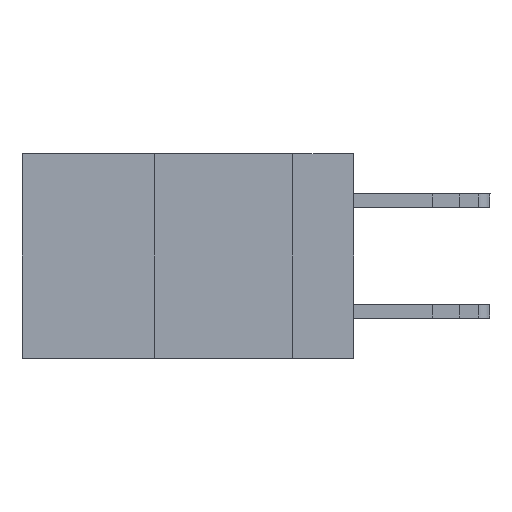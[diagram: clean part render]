
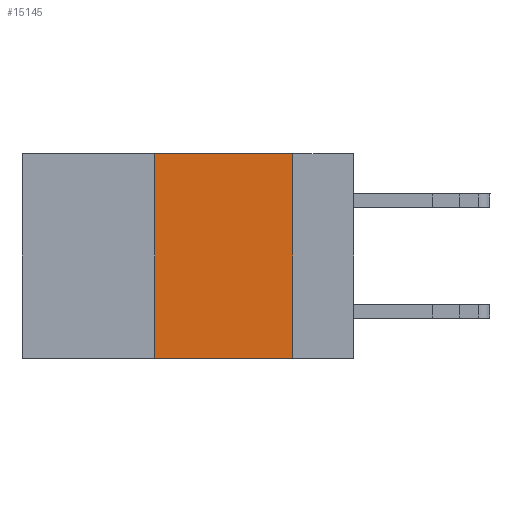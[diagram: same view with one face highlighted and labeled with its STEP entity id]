
A CAD part, left-side view. The second image highlights one B-rep face of the part: STEP entity #15145.
In plain terms, the highlighted planar face has unit normal (-1, 0, 0).
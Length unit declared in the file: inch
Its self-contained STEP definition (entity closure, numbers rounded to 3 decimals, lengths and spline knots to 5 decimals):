
#820 = DIRECTION ( 'NONE',  ( 0., 0., -1. ) ) ;
#977 = CARTESIAN_POINT ( 'NONE',  ( 0., 0.11, 0. ) ) ;
#1114 = VERTEX_POINT ( 'NONE', #13516 ) ;
#1533 = LINE ( 'NONE', #15673, #16303 ) ;
#2471 = CARTESIAN_POINT ( 'NONE',  ( 0., 0.6, -0.37 ) ) ;
#3147 = LINE ( 'NONE', #15863, #15089 ) ;
#6075 = ORIENTED_EDGE ( 'NONE', *, *, #16680, .F. ) ;
#6268 = FACE_OUTER_BOUND ( 'NONE', #8797, .T. ) ;
#7765 = VECTOR ( 'NONE', #22078, 39.37008 ) ;
#8781 = ORIENTED_EDGE ( 'NONE', *, *, #11999, .F. ) ;
#8797 = EDGE_LOOP ( 'NONE', ( #8781, #6075, #22035, #15753 ) ) ;
#9695 = VERTEX_POINT ( 'NONE', #977 ) ;
#10950 = LINE ( 'NONE', #2471, #13318 ) ;
#11747 = DIRECTION ( 'NONE',  ( 0., -1., 0. ) ) ;
#11999 = EDGE_CURVE ( 'NONE', #9695, #12107, #13712, .T. ) ;
#12107 = VERTEX_POINT ( 'NONE', #17070 ) ;
#13318 = VECTOR ( 'NONE', #16484, 39.37008 ) ;
#13516 = CARTESIAN_POINT ( 'NONE',  ( 0., 0.36, 0. ) ) ;
#13642 = VERTEX_POINT ( 'NONE', #20904 ) ;
#13712 = LINE ( 'NONE', #18902, #7765 ) ;
#14265 = EDGE_CURVE ( 'NONE', #13642, #1114, #3147, .T. ) ;
#14950 = DIRECTION ( 'NONE',  ( 1., 0., 0. ) ) ;
#15089 = VECTOR ( 'NONE', #16338, 39.37008 ) ;
#15126 = AXIS2_PLACEMENT_3D ( 'NONE', #16346, #14950, #820 ) ;
#15145 = ADVANCED_FACE ( 'NONE', ( #6268 ), #18162, .F. ) ;
#15673 = CARTESIAN_POINT ( 'NONE',  ( 0., 0.6, 0. ) ) ;
#15753 = ORIENTED_EDGE ( 'NONE', *, *, #16240, .T. ) ;
#15863 = CARTESIAN_POINT ( 'NONE',  ( 0., 0.36, 0. ) ) ;
#16240 = EDGE_CURVE ( 'NONE', #13642, #12107, #10950, .T. ) ;
#16303 = VECTOR ( 'NONE', #11747, 39.37008 ) ;
#16338 = DIRECTION ( 'NONE',  ( 0., 0., 1. ) ) ;
#16346 = CARTESIAN_POINT ( 'NONE',  ( 0., 0.6, 0. ) ) ;
#16484 = DIRECTION ( 'NONE',  ( 0., -1., 0. ) ) ;
#16680 = EDGE_CURVE ( 'NONE', #1114, #9695, #1533, .T. ) ;
#17070 = CARTESIAN_POINT ( 'NONE',  ( 0., 0.11, -0.37 ) ) ;
#18162 = PLANE ( 'NONE',  #15126 ) ;
#18902 = CARTESIAN_POINT ( 'NONE',  ( 0., 0.11, 0. ) ) ;
#20904 = CARTESIAN_POINT ( 'NONE',  ( 0., 0.36, -0.37 ) ) ;
#22035 = ORIENTED_EDGE ( 'NONE', *, *, #14265, .F. ) ;
#22078 = DIRECTION ( 'NONE',  ( 0., 0., -1. ) ) ;
